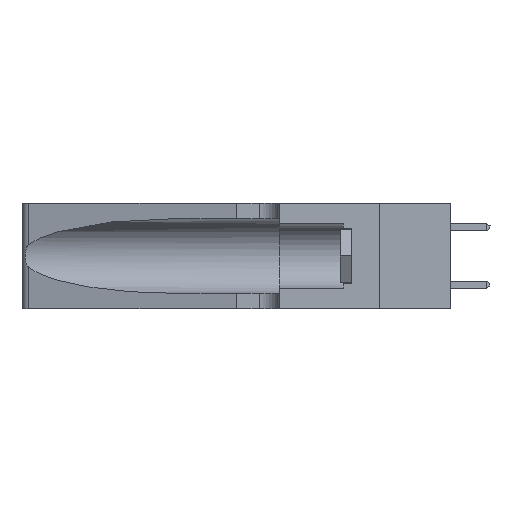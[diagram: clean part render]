
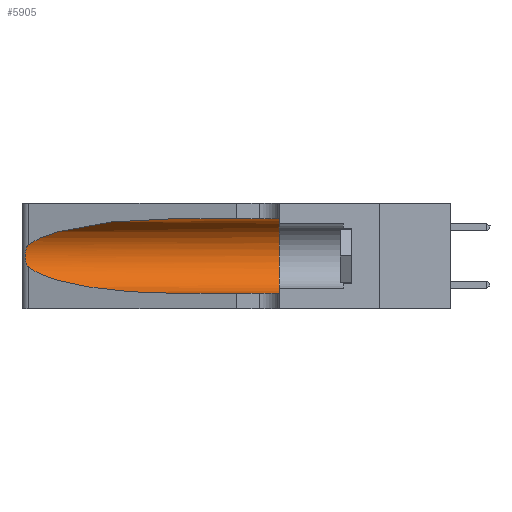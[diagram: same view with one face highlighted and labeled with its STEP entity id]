
A CAD part, left-side view. The second image highlights one B-rep face of the part: STEP entity #5905.
In plain terms, the highlighted cylindrical face has radius 3.308 mm (diameter 6.617 mm), a partial arc.
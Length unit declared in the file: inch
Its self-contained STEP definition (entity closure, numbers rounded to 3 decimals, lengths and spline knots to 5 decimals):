
#727 = CARTESIAN_POINT ( 'NONE',  ( 0.26075, 1.23896, 0.178 ) ) ;
#1383 = ORIENTED_EDGE ( 'NONE', *, *, #5394, .T. ) ;
#1557 = DIRECTION ( 'NONE',  ( 0., 1., 0. ) ) ;
#1994 = CARTESIAN_POINT ( 'NONE',  ( 0.25487, 1.22718, 0.22369 ) ) ;
#2113 = CARTESIAN_POINT ( 'NONE',  ( 0.25856, 1.23593, 0.16098 ) ) ;
#2169 = CARTESIAN_POINT ( 'NONE',  ( 0.1305, 1.61858, 0.185 ) ) ;
#3153 =( BOUNDED_CURVE ( )  B_SPLINE_CURVE ( 3, ( #6950, #12014, #5659, #15899 ),
 .UNSPECIFIED., .F., .F. ) 
 B_SPLINE_CURVE_WITH_KNOTS ( ( 4, 4 ),
 ( 1.5708, 2.84003 ),
 .UNSPECIFIED. ) 
 CURVE ( )  GEOMETRIC_REPRESENTATION_ITEM ( )  RATIONAL_B_SPLINE_CURVE ( ( 1., 0.87, 0.87, 1. ) ) 
 REPRESENTATION_ITEM ( '' )  );
#3165 = AXIS2_PLACEMENT_3D ( 'NONE', #9430, #1557, #10741 ) ;
#3213 = EDGE_CURVE ( 'NONE', #15638, #4767, #3153, .T. ) ;
#3429 = CARTESIAN_POINT ( 'NONE',  ( 0.25487, 1.22718, 0.22369 ) ) ;
#3488 = CARTESIAN_POINT ( 'NONE',  ( 0.25639, 1.23186, 0.15144 ) ) ;
#3914 = DIRECTION ( 'NONE',  ( 0., -1., 0. ) ) ;
#4120 = ORIENTED_EDGE ( 'NONE', *, *, #3213, .T. ) ;
#4130 = VERTEX_POINT ( 'NONE', #11281 ) ;
#4767 = VERTEX_POINT ( 'NONE', #1994 ) ;
#4848 = CARTESIAN_POINT ( 'NONE',  ( 0.25487, 1.22718, 0.14631 ) ) ;
#4973 = LINE ( 'NONE', #11650, #10992 ) ;
#5002 = EDGE_CURVE ( 'NONE', #15638, #14228, #4973, .T. ) ;
#5394 = EDGE_CURVE ( 'NONE', #4130, #10521, #14431, .T. ) ;
#5659 = CARTESIAN_POINT ( 'NONE',  ( 0.2373, 1.15595, 0.28018 ) ) ;
#5905 = ADVANCED_FACE ( 'NONE', ( #10781 ), #16812, .F. ) ;
#6122 = CARTESIAN_POINT ( 'NONE',  ( 0.25639, 1.23184, 0.21858 ) ) ;
#6177 = DIRECTION ( 'NONE',  ( 0., -1., 0. ) ) ;
#6717 = ORIENTED_EDGE ( 'NONE', *, *, #5002, .F. ) ;
#6940 = CARTESIAN_POINT ( 'NONE',  ( 0.1305, 0.35, 0.05475 ) ) ;
#6950 = CARTESIAN_POINT ( 'NONE',  ( 0.1305, 0.72297, 0.31525 ) ) ;
#7191 = VECTOR ( 'NONE', #10073, 39.37008 ) ;
#7402 = CARTESIAN_POINT ( 'NONE',  ( 0.25854, 1.2359, 0.20912 ) ) ;
#7417 = CARTESIAN_POINT ( 'NONE',  ( 0.1305, 0.72297, 0.05475 ) ) ;
#8124 = EDGE_LOOP ( 'NONE', ( #4120, #12699, #8421, #1383, #12765, #6717 ) ) ;
#8421 = ORIENTED_EDGE ( 'NONE', *, *, #9459, .T. ) ;
#8638 = CARTESIAN_POINT ( 'NONE',  ( 0.26075, 1.23896, 0.19203 ) ) ;
#8984 = CIRCLE ( 'NONE', #3165, 0.13025 ) ;
#9350 = CARTESIAN_POINT ( 'NONE',  ( 0.1305, 0.72297, 0.31525 ) ) ;
#9430 = CARTESIAN_POINT ( 'NONE',  ( 0.1305, 0.35, 0.185 ) ) ;
#9459 = EDGE_CURVE ( 'NONE', #13916, #4130, #10418, .T. ) ;
#9912 = CARTESIAN_POINT ( 'NONE',  ( 0.1305, 0.35, 0.31525 ) ) ;
#9968 = CARTESIAN_POINT ( 'NONE',  ( 0.26017, 1.23833, 0.17102 ) ) ;
#10026 = DIRECTION ( 'NONE',  ( 0., 0., -1. ) ) ;
#10073 = DIRECTION ( 'NONE',  ( 0., -1., 0. ) ) ;
#10418 =( BOUNDED_CURVE ( )  B_SPLINE_CURVE ( 3, ( #12523, #13809, #15108, #7417 ),
 .UNSPECIFIED., .F., .F. ) 
 B_SPLINE_CURVE_WITH_KNOTS ( ( 4, 4 ),
 ( 3.44316, 4.71239 ),
 .UNSPECIFIED. ) 
 CURVE ( )  GEOMETRIC_REPRESENTATION_ITEM ( )  RATIONAL_B_SPLINE_CURVE ( ( 1., 0.87, 0.87, 1. ) ) 
 REPRESENTATION_ITEM ( '' )  );
#10521 = VERTEX_POINT ( 'NONE', #6940 ) ;
#10741 = DIRECTION ( 'NONE',  ( 0., 0., 1. ) ) ;
#10781 = FACE_OUTER_BOUND ( 'NONE', #8124, .T. ) ;
#10992 = VECTOR ( 'NONE', #3914, 39.37008 ) ;
#11260 = CARTESIAN_POINT ( 'NONE',  ( 0.25789, 1.23486, 0.15765 ) ) ;
#11281 = CARTESIAN_POINT ( 'NONE',  ( 0.1305, 0.72297, 0.05475 ) ) ;
#11650 = CARTESIAN_POINT ( 'NONE',  ( 0.1305, 1.61858, 0.31525 ) ) ;
#11825 = B_SPLINE_CURVE_WITH_KNOTS ( 'NONE', 3,
 ( #3429, #13790, #6122, #15091, #7402, #16349, #8638, #727, #9968, #2113, #11260, #3488, #12557, #4848 ),
 .UNSPECIFIED., .F., .F.,
 ( 4, 2, 2, 2, 2, 2, 4 ),
 ( 0., 0.00027, 0.00053, 0.00107, 0.0016, 0.00187, 0.00214 ),
 .UNSPECIFIED. ) ;
#12014 = CARTESIAN_POINT ( 'NONE',  ( 0.18966, 0.96281, 0.31525 ) ) ;
#12164 = EDGE_CURVE ( 'NONE', #14228, #10521, #8984, .T. ) ;
#12337 = AXIS2_PLACEMENT_3D ( 'NONE', #2169, #6177, #10026 ) ;
#12523 = CARTESIAN_POINT ( 'NONE',  ( 0.25487, 1.22718, 0.14631 ) ) ;
#12557 = CARTESIAN_POINT ( 'NONE',  ( 0.25555, 1.22993, 0.14849 ) ) ;
#12699 = ORIENTED_EDGE ( 'NONE', *, *, #14229, .T. ) ;
#12765 = ORIENTED_EDGE ( 'NONE', *, *, #12164, .F. ) ;
#13790 = CARTESIAN_POINT ( 'NONE',  ( 0.25555, 1.22994, 0.2215 ) ) ;
#13809 = CARTESIAN_POINT ( 'NONE',  ( 0.2373, 1.15595, 0.08982 ) ) ;
#13916 = VERTEX_POINT ( 'NONE', #14388 ) ;
#14228 = VERTEX_POINT ( 'NONE', #9912 ) ;
#14229 = EDGE_CURVE ( 'NONE', #4767, #13916, #11825, .T. ) ;
#14388 = CARTESIAN_POINT ( 'NONE',  ( 0.25487, 1.22718, 0.14631 ) ) ;
#14431 = LINE ( 'NONE', #16446, #7191 ) ;
#15091 = CARTESIAN_POINT ( 'NONE',  ( 0.25787, 1.23484, 0.2124 ) ) ;
#15108 = CARTESIAN_POINT ( 'NONE',  ( 0.18966, 0.96281, 0.05475 ) ) ;
#15638 = VERTEX_POINT ( 'NONE', #9350 ) ;
#15899 = CARTESIAN_POINT ( 'NONE',  ( 0.25487, 1.22718, 0.22369 ) ) ;
#16349 = CARTESIAN_POINT ( 'NONE',  ( 0.26018, 1.23835, 0.19895 ) ) ;
#16446 = CARTESIAN_POINT ( 'NONE',  ( 0.1305, 1.61858, 0.05475 ) ) ;
#16812 = CYLINDRICAL_SURFACE ( 'NONE', #12337, 0.13025 ) ;
